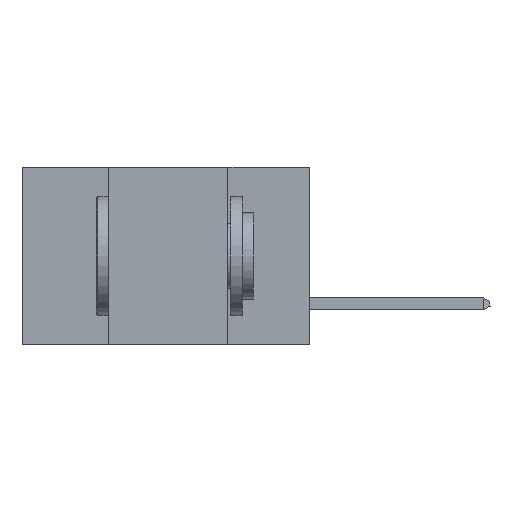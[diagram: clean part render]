
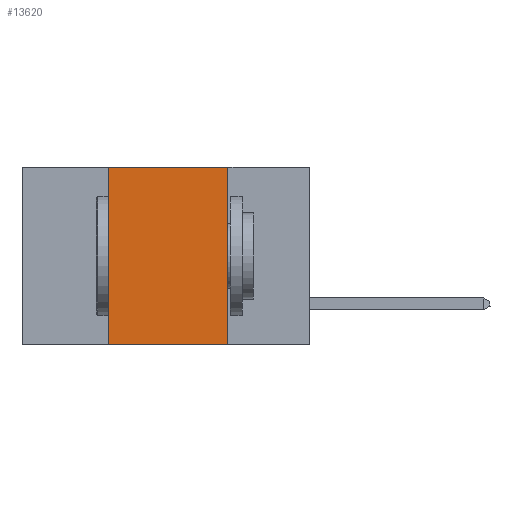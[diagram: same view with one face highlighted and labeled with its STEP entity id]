
A CAD part, left-side view. The second image highlights one B-rep face of the part: STEP entity #13620.
In plain terms, the highlighted planar face has unit normal (-1, 0, 0).
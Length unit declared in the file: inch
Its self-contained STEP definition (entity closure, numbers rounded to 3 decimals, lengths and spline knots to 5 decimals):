
#122 = ORIENTED_EDGE ( 'NONE', *, *, #15126, .F. ) ;
#2058 = CARTESIAN_POINT ( 'NONE',  ( 0., 0.42, -0.37 ) ) ;
#2582 = CARTESIAN_POINT ( 'NONE',  ( 0., 0.17, 0. ) ) ;
#2719 = CARTESIAN_POINT ( 'NONE',  ( 0., 0.42, 0. ) ) ;
#3668 = DIRECTION ( 'NONE',  ( 0., 0., 1. ) ) ;
#3819 = VERTEX_POINT ( 'NONE', #5033 ) ;
#4066 = EDGE_LOOP ( 'NONE', ( #122, #17374, #6678, #13449 ) ) ;
#4134 = VERTEX_POINT ( 'NONE', #2719 ) ;
#4557 = CARTESIAN_POINT ( 'NONE',  ( 0., 0.17, 0. ) ) ;
#4816 = EDGE_CURVE ( 'NONE', #5259, #3819, #15661, .T. ) ;
#5026 = LINE ( 'NONE', #28616, #11218 ) ;
#5033 = CARTESIAN_POINT ( 'NONE',  ( 0., 0.17, -0.37 ) ) ;
#5103 = CARTESIAN_POINT ( 'NONE',  ( 0., 0.6, -0.37 ) ) ;
#5105 = CARTESIAN_POINT ( 'NONE',  ( 0., 0.6, 0. ) ) ;
#5259 = VERTEX_POINT ( 'NONE', #2058 ) ;
#5274 = VECTOR ( 'NONE', #11202, 39.37008 ) ;
#6678 = ORIENTED_EDGE ( 'NONE', *, *, #26195, .F. ) ;
#7398 = DIRECTION ( 'NONE',  ( 0., -1., 0. ) ) ;
#8757 = FACE_OUTER_BOUND ( 'NONE', #4066, .T. ) ;
#11202 = DIRECTION ( 'NONE',  ( 0., 0., -1. ) ) ;
#11218 = VECTOR ( 'NONE', #22750, 39.37008 ) ;
#11273 = PLANE ( 'NONE',  #23372 ) ;
#11498 = LINE ( 'NONE', #4557, #5274 ) ;
#13449 = ORIENTED_EDGE ( 'NONE', *, *, #4816, .T. ) ;
#13620 = ADVANCED_FACE ( 'NONE', ( #8757 ), #11273, .F. ) ;
#14721 = LINE ( 'NONE', #23307, #22287 ) ;
#14991 = VECTOR ( 'NONE', #7398, 39.37008 ) ;
#15126 = EDGE_CURVE ( 'NONE', #26047, #3819, #11498, .T. ) ;
#15661 = LINE ( 'NONE', #5103, #14991 ) ;
#17374 = ORIENTED_EDGE ( 'NONE', *, *, #25480, .F. ) ;
#22287 = VECTOR ( 'NONE', #3668, 39.37008 ) ;
#22705 = DIRECTION ( 'NONE',  ( 1., 0., 0. ) ) ;
#22750 = DIRECTION ( 'NONE',  ( 0., -1., 0. ) ) ;
#23307 = CARTESIAN_POINT ( 'NONE',  ( 0., 0.42, 0. ) ) ;
#23372 = AXIS2_PLACEMENT_3D ( 'NONE', #5105, #22705, #26887 ) ;
#25480 = EDGE_CURVE ( 'NONE', #4134, #26047, #5026, .T. ) ;
#26047 = VERTEX_POINT ( 'NONE', #2582 ) ;
#26195 = EDGE_CURVE ( 'NONE', #5259, #4134, #14721, .T. ) ;
#26887 = DIRECTION ( 'NONE',  ( 0., 0., -1. ) ) ;
#28616 = CARTESIAN_POINT ( 'NONE',  ( 0., 0.6, 0. ) ) ;
